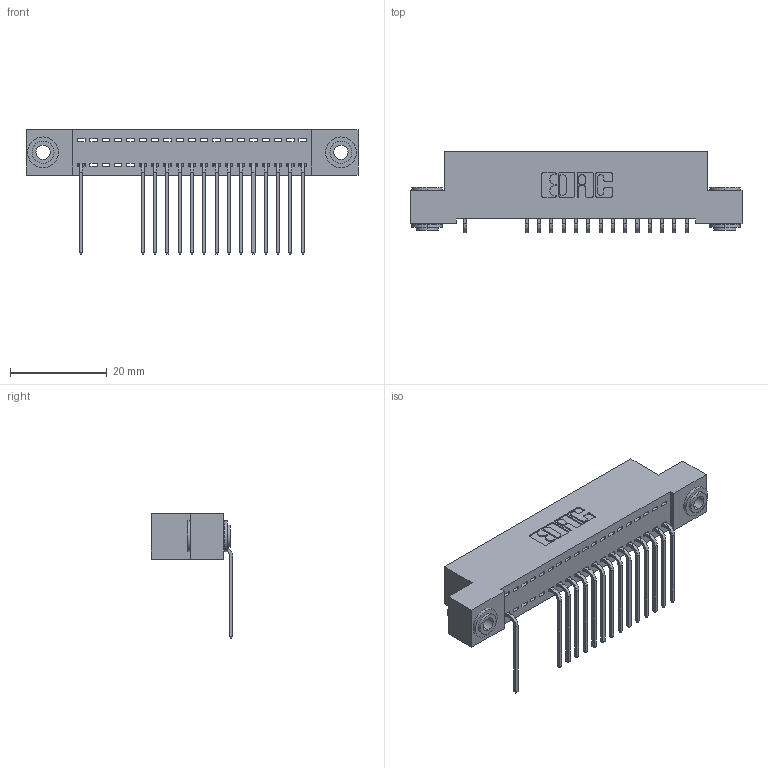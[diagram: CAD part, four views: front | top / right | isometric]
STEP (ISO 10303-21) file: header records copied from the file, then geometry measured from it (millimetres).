
FILE_DESCRIPTION (( 'STEP AP203' ), '1' );
FILE_NAME ('392-019-559-103.STEP', '2018-08-15T05:46:05', ( '' ), ( '' ), 'SwSTEP 2.0', 'SolidWorks 2016', '' );
FILE_SCHEMA (( 'CONFIG_CONTROL_DESIGN' ));
Length unit declared in the file: inch
Products named in the file (4): 342 Part_.156 TH; 345-292-001_558 559 Tail - 1; 342-250-002_345-250-002-102; 392-019-559-103
Assembly tree (18 placements, depth 2):
  392-019-559-103
    342 Part_.156 TH
    345-292-001_558 559 Tail - 1  x15
    342-250-002_345-250-002-102  x2
Bounding box: 68.58 x 16.83 x 25.78 mm (x, y, z)
Volume: 5955.4 mm3; surface area: 8588.8 mm2
Topology: 18 solids, 18 shells, 1096 faces, 3273 edges, 2158 vertices
Faces by surface type: plane 784, cylinder 304, cone 8
Entity records: 15064 total; most frequent: CARTESIAN_POINT 2598, ORIENTED_EDGE 2550, DIRECTION 2267, EDGE_CURVE 1275, LINE 1123, VECTOR 1123, VERTEX_POINT 846, AXIS2_PLACEMENT_3D 572
